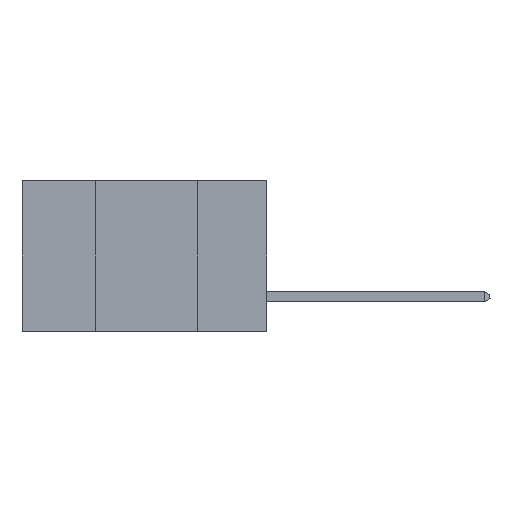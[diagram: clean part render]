
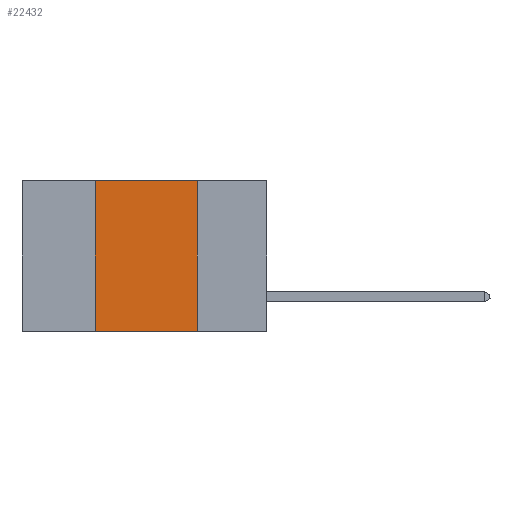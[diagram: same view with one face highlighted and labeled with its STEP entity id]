
A CAD part, left-side view. The second image highlights one B-rep face of the part: STEP entity #22432.
In plain terms, the highlighted planar face has unit normal (-1, 0, 0).
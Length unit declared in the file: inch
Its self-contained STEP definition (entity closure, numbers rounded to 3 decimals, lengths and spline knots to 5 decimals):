
#3222 = DIRECTION ( 'NONE',  ( 0., -1., 0. ) ) ;
#5657 = CARTESIAN_POINT ( 'NONE',  ( 0., 0.42, 0. ) ) ;
#6028 = LINE ( 'NONE', #22879, #13849 ) ;
#7404 = VECTOR ( 'NONE', #9409, 39.37008 ) ;
#8739 = VECTOR ( 'NONE', #18528, 39.37008 ) ;
#9112 = EDGE_CURVE ( 'NONE', #9613, #10884, #16957, .T. ) ;
#9133 = PLANE ( 'NONE',  #21798 ) ;
#9409 = DIRECTION ( 'NONE',  ( 0., 0., 1. ) ) ;
#9613 = VERTEX_POINT ( 'NONE', #10827 ) ;
#10344 = VECTOR ( 'NONE', #10854, 39.37008 ) ;
#10750 = CARTESIAN_POINT ( 'NONE',  ( 0., 0.17, -0.37 ) ) ;
#10827 = CARTESIAN_POINT ( 'NONE',  ( 0., 0.42, -0.37 ) ) ;
#10854 = DIRECTION ( 'NONE',  ( 0., -1., 0. ) ) ;
#10884 = VERTEX_POINT ( 'NONE', #10750 ) ;
#11631 = DIRECTION ( 'NONE',  ( 0., 0., -1. ) ) ;
#13364 = VERTEX_POINT ( 'NONE', #14188 ) ;
#13849 = VECTOR ( 'NONE', #3222, 39.37008 ) ;
#14188 = CARTESIAN_POINT ( 'NONE',  ( 0., 0.17, 0. ) ) ;
#14630 = ORIENTED_EDGE ( 'NONE', *, *, #9112, .T. ) ;
#16309 = CARTESIAN_POINT ( 'NONE',  ( 0., 0.6, 0. ) ) ;
#16524 = DIRECTION ( 'NONE',  ( 1., 0., 0. ) ) ;
#16957 = LINE ( 'NONE', #28082, #10344 ) ;
#18528 = DIRECTION ( 'NONE',  ( 0., 0., -1. ) ) ;
#19530 = EDGE_LOOP ( 'NONE', ( #22075, #30147, #21462, #14630 ) ) ;
#21353 = EDGE_CURVE ( 'NONE', #9613, #21540, #23825, .T. ) ;
#21462 = ORIENTED_EDGE ( 'NONE', *, *, #21353, .F. ) ;
#21540 = VERTEX_POINT ( 'NONE', #5657 ) ;
#21798 = AXIS2_PLACEMENT_3D ( 'NONE', #16309, #16524, #11631 ) ;
#22000 = LINE ( 'NONE', #23560, #8739 ) ;
#22075 = ORIENTED_EDGE ( 'NONE', *, *, #29091, .F. ) ;
#22432 = ADVANCED_FACE ( 'NONE', ( #30715 ), #9133, .F. ) ;
#22879 = CARTESIAN_POINT ( 'NONE',  ( 0., 0.6, 0. ) ) ;
#23560 = CARTESIAN_POINT ( 'NONE',  ( 0., 0.17, 0. ) ) ;
#23729 = EDGE_CURVE ( 'NONE', #21540, #13364, #6028, .T. ) ;
#23825 = LINE ( 'NONE', #31847, #7404 ) ;
#28082 = CARTESIAN_POINT ( 'NONE',  ( 0., 0.6, -0.37 ) ) ;
#29091 = EDGE_CURVE ( 'NONE', #13364, #10884, #22000, .T. ) ;
#30147 = ORIENTED_EDGE ( 'NONE', *, *, #23729, .F. ) ;
#30715 = FACE_OUTER_BOUND ( 'NONE', #19530, .T. ) ;
#31847 = CARTESIAN_POINT ( 'NONE',  ( 0., 0.42, 0. ) ) ;
